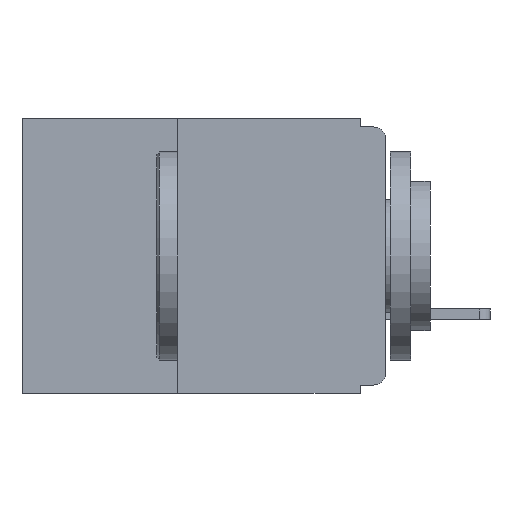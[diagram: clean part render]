
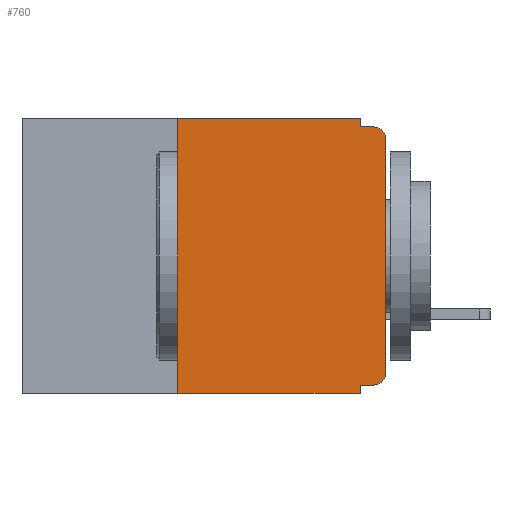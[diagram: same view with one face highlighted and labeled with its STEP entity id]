
A CAD part, left-side view. The second image highlights one B-rep face of the part: STEP entity #760.
In plain terms, the highlighted planar face has unit normal (-1, 0, 0).
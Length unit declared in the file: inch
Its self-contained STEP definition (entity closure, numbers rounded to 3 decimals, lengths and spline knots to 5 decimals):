
#209 = DIRECTION ( 'NONE',  ( 0., 0., -1. ) ) ;
#356 = LINE ( 'NONE', #482, #10660 ) ;
#402 = ORIENTED_EDGE ( 'NONE', *, *, #8711, .F. ) ;
#482 = CARTESIAN_POINT ( 'NONE',  ( 0., 0.031, 0. ) ) ;
#566 = LINE ( 'NONE', #12286, #10863 ) ;
#760 = ADVANCED_FACE ( 'NONE', ( #25937 ), #3555, .F. ) ;
#1670 = CARTESIAN_POINT ( 'NONE',  ( 0., 0.015, -0.01 ) ) ;
#1909 = DIRECTION ( 'NONE',  ( 0., 0., 1. ) ) ;
#2521 = ORIENTED_EDGE ( 'NONE', *, *, #20728, .T. ) ;
#2538 = DIRECTION ( 'NONE',  ( 0., 0., -1. ) ) ;
#2991 = VERTEX_POINT ( 'NONE', #13104 ) ;
#3555 = PLANE ( 'NONE',  #24566 ) ;
#3726 = VECTOR ( 'NONE', #15155, 39.37008 ) ;
#3833 = EDGE_CURVE ( 'NONE', #17776, #3974, #24028, .T. ) ;
#3974 = VERTEX_POINT ( 'NONE', #1670 ) ;
#4144 = DIRECTION ( 'NONE',  ( 1., 0., 0. ) ) ;
#4376 = CARTESIAN_POINT ( 'NONE',  ( 0., 0., -0.01 ) ) ;
#4426 = DIRECTION ( 'NONE',  ( 0., -1., 0. ) ) ;
#4642 = VECTOR ( 'NONE', #1909, 39.37008 ) ;
#4994 = EDGE_CURVE ( 'NONE', #11542, #21448, #566, .T. ) ;
#6126 = ORIENTED_EDGE ( 'NONE', *, *, #3833, .F. ) ;
#6149 = EDGE_CURVE ( 'NONE', #9666, #11854, #19479, .T. ) ;
#7079 = ORIENTED_EDGE ( 'NONE', *, *, #24158, .T. ) ;
#7101 = CARTESIAN_POINT ( 'NONE',  ( 0., 0.015, -0.025 ) ) ;
#7330 = CARTESIAN_POINT ( 'NONE',  ( 0., 0.437, 0. ) ) ;
#7551 = EDGE_LOOP ( 'NONE', ( #2521, #7079, #6126, #25611, #26242, #18053, #19365, #22539, #402, #11961 ) ) ;
#7892 = CARTESIAN_POINT ( 'NONE',  ( 0., 0.031, -0.01 ) ) ;
#8351 = CARTESIAN_POINT ( 'NONE',  ( 0., 0.437, -0.33 ) ) ;
#8711 = EDGE_CURVE ( 'NONE', #16860, #11542, #22053, .T. ) ;
#8958 = CARTESIAN_POINT ( 'NONE',  ( 0., 0.031, -0.32 ) ) ;
#9154 = DIRECTION ( 'NONE',  ( 0., 0., -1. ) ) ;
#9185 = CARTESIAN_POINT ( 'NONE',  ( 0., 0.031, -0.33 ) ) ;
#9666 = VERTEX_POINT ( 'NONE', #17335 ) ;
#9938 = VECTOR ( 'NONE', #24687, 39.37008 ) ;
#10131 = LINE ( 'NONE', #26402, #4642 ) ;
#10660 = VECTOR ( 'NONE', #2538, 39.37008 ) ;
#10863 = VECTOR ( 'NONE', #12218, 39.37008 ) ;
#11542 = VERTEX_POINT ( 'NONE', #8958 ) ;
#11737 = DIRECTION ( 'NONE',  ( 0., 0., -1. ) ) ;
#11854 = VERTEX_POINT ( 'NONE', #24316 ) ;
#11961 = ORIENTED_EDGE ( 'NONE', *, *, #13717, .T. ) ;
#12218 = DIRECTION ( 'NONE',  ( 0., 0., -1. ) ) ;
#12286 = CARTESIAN_POINT ( 'NONE',  ( 0., 0.031, -0.33 ) ) ;
#12507 = DIRECTION ( 'NONE',  ( -1., 0., 0. ) ) ;
#13104 = CARTESIAN_POINT ( 'NONE',  ( 0., 0.031, 0. ) ) ;
#13717 = EDGE_CURVE ( 'NONE', #16860, #16365, #16412, .T. ) ;
#15155 = DIRECTION ( 'NONE',  ( 0., 0., 1. ) ) ;
#15180 = CARTESIAN_POINT ( 'NONE',  ( 0., 0.25, -0.33 ) ) ;
#15474 = EDGE_CURVE ( 'NONE', #9666, #21448, #26180, .T. ) ;
#16343 = AXIS2_PLACEMENT_3D ( 'NONE', #24749, #12507, #209 ) ;
#16365 = VERTEX_POINT ( 'NONE', #25703 ) ;
#16412 = CIRCLE ( 'NONE', #16343, 0.015 ) ;
#16654 = VECTOR ( 'NONE', #22449, 39.37008 ) ;
#16860 = VERTEX_POINT ( 'NONE', #23121 ) ;
#17335 = CARTESIAN_POINT ( 'NONE',  ( 0., 0.25, -0.33 ) ) ;
#17776 = VERTEX_POINT ( 'NONE', #7892 ) ;
#18053 = ORIENTED_EDGE ( 'NONE', *, *, #6149, .F. ) ;
#18670 = VECTOR ( 'NONE', #4426, 39.37008 ) ;
#19182 = LINE ( 'NONE', #22129, #23277 ) ;
#19365 = ORIENTED_EDGE ( 'NONE', *, *, #15474, .T. ) ;
#19479 = LINE ( 'NONE', #15180, #3726 ) ;
#19539 = EDGE_CURVE ( 'NONE', #11854, #2991, #19182, .T. ) ;
#20522 = CIRCLE ( 'NONE', #25212, 0.015 ) ;
#20728 = EDGE_CURVE ( 'NONE', #16365, #24293, #10131, .T. ) ;
#21413 = DIRECTION ( 'NONE',  ( -1., 0., 0. ) ) ;
#21448 = VERTEX_POINT ( 'NONE', #9185 ) ;
#22053 = LINE ( 'NONE', #24386, #16654 ) ;
#22129 = CARTESIAN_POINT ( 'NONE',  ( 0., 0.437, 0. ) ) ;
#22449 = DIRECTION ( 'NONE',  ( 0., 1., 0. ) ) ;
#22539 = ORIENTED_EDGE ( 'NONE', *, *, #4994, .F. ) ;
#23058 = EDGE_CURVE ( 'NONE', #2991, #17776, #356, .T. ) ;
#23121 = CARTESIAN_POINT ( 'NONE',  ( 0., 0.015, -0.32 ) ) ;
#23277 = VECTOR ( 'NONE', #24163, 39.37008 ) ;
#24028 = LINE ( 'NONE', #4376, #18670 ) ;
#24158 = EDGE_CURVE ( 'NONE', #24293, #3974, #20522, .T. ) ;
#24163 = DIRECTION ( 'NONE',  ( 0., -1., 0. ) ) ;
#24293 = VERTEX_POINT ( 'NONE', #25832 ) ;
#24316 = CARTESIAN_POINT ( 'NONE',  ( 0., 0.25, 0. ) ) ;
#24386 = CARTESIAN_POINT ( 'NONE',  ( 0., 0., -0.32 ) ) ;
#24566 = AXIS2_PLACEMENT_3D ( 'NONE', #7330, #4144, #11737 ) ;
#24687 = DIRECTION ( 'NONE',  ( 0., -1., 0. ) ) ;
#24749 = CARTESIAN_POINT ( 'NONE',  ( 0., 0.015, -0.305 ) ) ;
#25212 = AXIS2_PLACEMENT_3D ( 'NONE', #7101, #21413, #9154 ) ;
#25611 = ORIENTED_EDGE ( 'NONE', *, *, #23058, .F. ) ;
#25703 = CARTESIAN_POINT ( 'NONE',  ( 0., 0., -0.305 ) ) ;
#25832 = CARTESIAN_POINT ( 'NONE',  ( 0., 0., -0.025 ) ) ;
#25937 = FACE_OUTER_BOUND ( 'NONE', #7551, .T. ) ;
#26180 = LINE ( 'NONE', #8351, #9938 ) ;
#26242 = ORIENTED_EDGE ( 'NONE', *, *, #19539, .F. ) ;
#26402 = CARTESIAN_POINT ( 'NONE',  ( 0., 0., 0. ) ) ;
